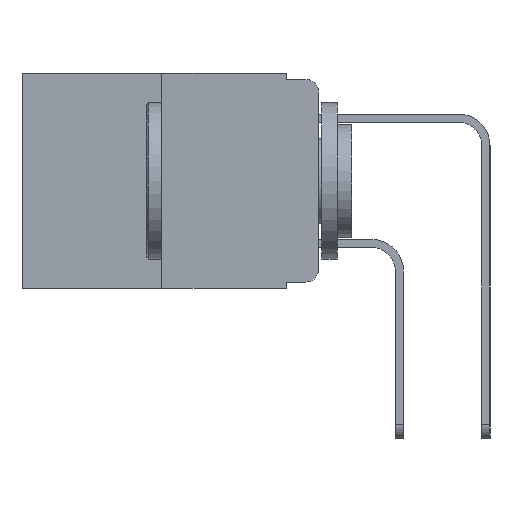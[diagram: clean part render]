
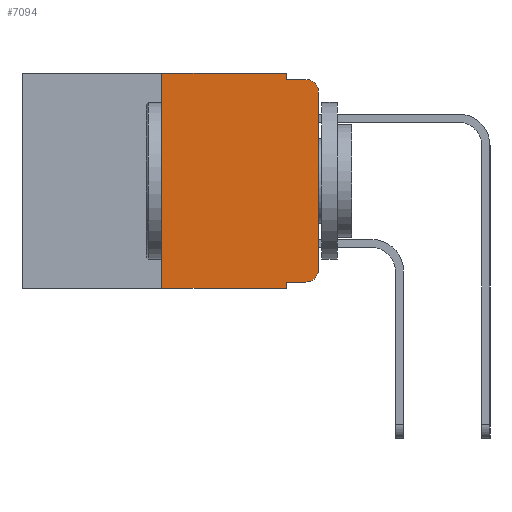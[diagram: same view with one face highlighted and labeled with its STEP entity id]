
A CAD part, left-side view. The second image highlights one B-rep face of the part: STEP entity #7094.
In plain terms, the highlighted planar face has unit normal (-1, 0, 0).
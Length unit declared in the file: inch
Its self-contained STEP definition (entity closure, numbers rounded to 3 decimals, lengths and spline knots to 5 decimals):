
#77 = VERTEX_POINT ( 'NONE', #12101 ) ;
#164 = ORIENTED_EDGE ( 'NONE', *, *, #2008, .F. ) ;
#339 = ORIENTED_EDGE ( 'NONE', *, *, #2144, .T. ) ;
#539 = CARTESIAN_POINT ( 'NONE',  ( 0., 0.051, -0.333 ) ) ;
#653 = DIRECTION ( 'NONE',  ( -1., 0., 0. ) ) ;
#800 = VECTOR ( 'NONE', #7150, 39.37008 ) ;
#813 = CARTESIAN_POINT ( 'NONE',  ( 0., 0.02, -0.313 ) ) ;
#1234 = VECTOR ( 'NONE', #2522, 39.37008 ) ;
#1261 = VERTEX_POINT ( 'NONE', #9017 ) ;
#1267 = VERTEX_POINT ( 'NONE', #6635 ) ;
#1385 = VECTOR ( 'NONE', #1627, 39.37008 ) ;
#1423 = CARTESIAN_POINT ( 'NONE',  ( 0., 0.02, -0.01 ) ) ;
#1627 = DIRECTION ( 'NONE',  ( 0., 0., -1. ) ) ;
#1859 = ORIENTED_EDGE ( 'NONE', *, *, #3271, .F. ) ;
#1945 = CARTESIAN_POINT ( 'NONE',  ( 0., 0., 0. ) ) ;
#2008 = EDGE_CURVE ( 'NONE', #1261, #5593, #7340, .T. ) ;
#2009 = VECTOR ( 'NONE', #7869, 39.37008 ) ;
#2094 = CARTESIAN_POINT ( 'NONE',  ( 0., 0.473, 0. ) ) ;
#2144 = EDGE_CURVE ( 'NONE', #10322, #2872, #3764, .T. ) ;
#2151 = DIRECTION ( 'NONE',  ( 0., 0., -1. ) ) ;
#2180 = ORIENTED_EDGE ( 'NONE', *, *, #6870, .T. ) ;
#2303 = DIRECTION ( 'NONE',  ( 1., 0., 0. ) ) ;
#2343 = CARTESIAN_POINT ( 'NONE',  ( 0., 0., -0.03 ) ) ;
#2522 = DIRECTION ( 'NONE',  ( 0., 0., 1. ) ) ;
#2807 = LINE ( 'NONE', #11125, #8056 ) ;
#2872 = VERTEX_POINT ( 'NONE', #6390 ) ;
#2941 = CIRCLE ( 'NONE', #3879, 0.02 ) ;
#3139 = ORIENTED_EDGE ( 'NONE', *, *, #7821, .T. ) ;
#3271 = EDGE_CURVE ( 'NONE', #9173, #77, #3575, .T. ) ;
#3378 = CARTESIAN_POINT ( 'NONE',  ( 0., 0.473, -0.343 ) ) ;
#3575 = LINE ( 'NONE', #6540, #800 ) ;
#3614 = VECTOR ( 'NONE', #10168, 39.37008 ) ;
#3764 = CIRCLE ( 'NONE', #10965, 0.02 ) ;
#3879 = AXIS2_PLACEMENT_3D ( 'NONE', #4237, #10964, #5237 ) ;
#4135 = CARTESIAN_POINT ( 'NONE',  ( 0., 0.051, 0. ) ) ;
#4237 = CARTESIAN_POINT ( 'NONE',  ( 0., 0.02, -0.03 ) ) ;
#4247 = AXIS2_PLACEMENT_3D ( 'NONE', #2094, #2303, #9169 ) ;
#4417 = CARTESIAN_POINT ( 'NONE',  ( 0., 0.25, 0. ) ) ;
#4648 = VERTEX_POINT ( 'NONE', #6938 ) ;
#4956 = VERTEX_POINT ( 'NONE', #1423 ) ;
#5237 = DIRECTION ( 'NONE',  ( 0., 0., -1. ) ) ;
#5408 = DIRECTION ( 'NONE',  ( 0., -1., 0. ) ) ;
#5593 = VERTEX_POINT ( 'NONE', #4135 ) ;
#5707 = CARTESIAN_POINT ( 'NONE',  ( 0., 0.473, 0. ) ) ;
#5909 = DIRECTION ( 'NONE',  ( 0., -1., 0. ) ) ;
#6343 = LINE ( 'NONE', #4417, #1234 ) ;
#6390 = CARTESIAN_POINT ( 'NONE',  ( 0., 0., -0.313 ) ) ;
#6436 = ORIENTED_EDGE ( 'NONE', *, *, #12463, .T. ) ;
#6540 = CARTESIAN_POINT ( 'NONE',  ( 0., 0.051, 0. ) ) ;
#6634 = EDGE_LOOP ( 'NONE', ( #3139, #6436, #12032, #12334, #164, #11001, #8829, #1859, #2180, #339 ) ) ;
#6635 = CARTESIAN_POINT ( 'NONE',  ( 0., 0.051, -0.01 ) ) ;
#6639 = VECTOR ( 'NONE', #11403, 39.37008 ) ;
#6870 = EDGE_CURVE ( 'NONE', #9173, #10322, #10083, .T. ) ;
#6938 = CARTESIAN_POINT ( 'NONE',  ( 0., 0.25, -0.343 ) ) ;
#6988 = PLANE ( 'NONE',  #4247 ) ;
#7094 = ADVANCED_FACE ( 'NONE', ( #7739 ), #6988, .F. ) ;
#7150 = DIRECTION ( 'NONE',  ( 0., 0., -1. ) ) ;
#7340 = LINE ( 'NONE', #5707, #2009 ) ;
#7739 = FACE_OUTER_BOUND ( 'NONE', #6634, .T. ) ;
#7821 = EDGE_CURVE ( 'NONE', #2872, #9581, #11937, .T. ) ;
#7869 = DIRECTION ( 'NONE',  ( 0., -1., 0. ) ) ;
#7936 = LINE ( 'NONE', #3378, #3614 ) ;
#8056 = VECTOR ( 'NONE', #5408, 39.37008 ) ;
#8543 = EDGE_CURVE ( 'NONE', #4648, #1261, #6343, .T. ) ;
#8829 = ORIENTED_EDGE ( 'NONE', *, *, #10774, .T. ) ;
#9017 = CARTESIAN_POINT ( 'NONE',  ( 0., 0.25, 0. ) ) ;
#9143 = EDGE_CURVE ( 'NONE', #5593, #1267, #9580, .T. ) ;
#9169 = DIRECTION ( 'NONE',  ( 0., 0., -1. ) ) ;
#9173 = VERTEX_POINT ( 'NONE', #539 ) ;
#9580 = LINE ( 'NONE', #10426, #1385 ) ;
#9581 = VERTEX_POINT ( 'NONE', #2343 ) ;
#10083 = LINE ( 'NONE', #10554, #11987 ) ;
#10168 = DIRECTION ( 'NONE',  ( 0., -1., 0. ) ) ;
#10322 = VERTEX_POINT ( 'NONE', #12223 ) ;
#10426 = CARTESIAN_POINT ( 'NONE',  ( 0., 0.051, 0. ) ) ;
#10554 = CARTESIAN_POINT ( 'NONE',  ( 0., 0.051, -0.333 ) ) ;
#10774 = EDGE_CURVE ( 'NONE', #4648, #77, #7936, .T. ) ;
#10964 = DIRECTION ( 'NONE',  ( -1., 0., 0. ) ) ;
#10965 = AXIS2_PLACEMENT_3D ( 'NONE', #813, #653, #2151 ) ;
#11001 = ORIENTED_EDGE ( 'NONE', *, *, #8543, .F. ) ;
#11125 = CARTESIAN_POINT ( 'NONE',  ( 0., 0.051, -0.01 ) ) ;
#11403 = DIRECTION ( 'NONE',  ( 0., 0., 1. ) ) ;
#11429 = EDGE_CURVE ( 'NONE', #1267, #4956, #2807, .T. ) ;
#11937 = LINE ( 'NONE', #1945, #6639 ) ;
#11987 = VECTOR ( 'NONE', #5909, 39.37008 ) ;
#12032 = ORIENTED_EDGE ( 'NONE', *, *, #11429, .F. ) ;
#12101 = CARTESIAN_POINT ( 'NONE',  ( 0., 0.051, -0.343 ) ) ;
#12223 = CARTESIAN_POINT ( 'NONE',  ( 0., 0.02, -0.333 ) ) ;
#12334 = ORIENTED_EDGE ( 'NONE', *, *, #9143, .F. ) ;
#12463 = EDGE_CURVE ( 'NONE', #9581, #4956, #2941, .T. ) ;
